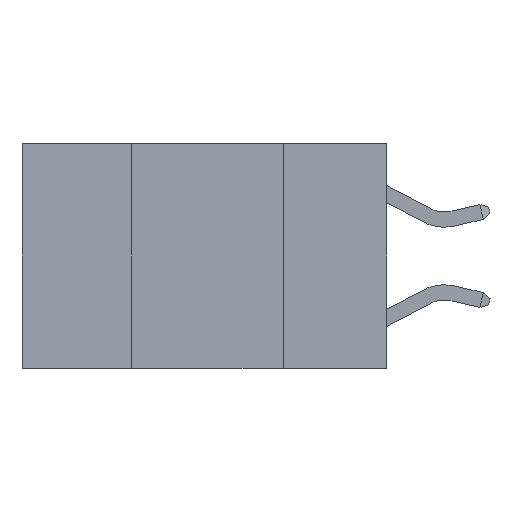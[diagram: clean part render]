
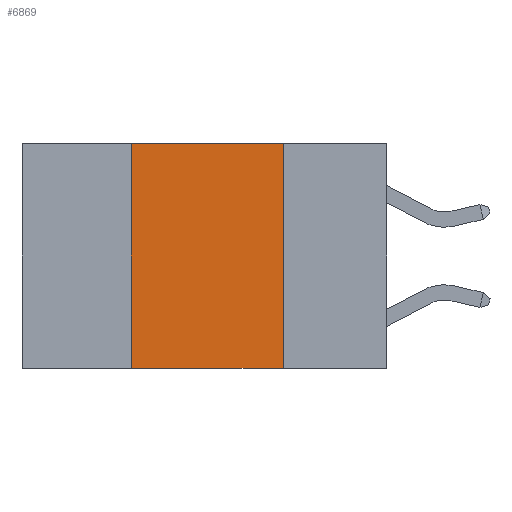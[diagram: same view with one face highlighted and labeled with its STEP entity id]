
A CAD part, left-side view. The second image highlights one B-rep face of the part: STEP entity #6869.
In plain terms, the highlighted planar face has unit normal (-1, 0, 0).
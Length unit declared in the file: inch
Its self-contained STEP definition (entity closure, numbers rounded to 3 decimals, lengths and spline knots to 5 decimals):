
#257 = FACE_OUTER_BOUND ( 'NONE', #26321, .T. ) ;
#2270 = LINE ( 'NONE', #10464, #5793 ) ;
#2395 = DIRECTION ( 'NONE',  ( 0., 0., -1. ) ) ;
#3506 = VECTOR ( 'NONE', #7858, 39.37008 ) ;
#3739 = EDGE_CURVE ( 'NONE', #3826, #25914, #2270, .T. ) ;
#3826 = VERTEX_POINT ( 'NONE', #24361 ) ;
#4052 = VERTEX_POINT ( 'NONE', #20062 ) ;
#4440 = DIRECTION ( 'NONE',  ( 0., 0., -1. ) ) ;
#5376 = CARTESIAN_POINT ( 'NONE',  ( 0., 0.42, 0. ) ) ;
#5665 = AXIS2_PLACEMENT_3D ( 'NONE', #24819, #14282, #4440 ) ;
#5793 = VECTOR ( 'NONE', #2395, 39.37008 ) ;
#6097 = ORIENTED_EDGE ( 'NONE', *, *, #3739, .F. ) ;
#6441 = PLANE ( 'NONE',  #5665 ) ;
#6869 = ADVANCED_FACE ( 'NONE', ( #257 ), #6441, .F. ) ;
#6937 = DIRECTION ( 'NONE',  ( 0., 0., 1. ) ) ;
#7195 = ORIENTED_EDGE ( 'NONE', *, *, #24867, .T. ) ;
#7238 = ORIENTED_EDGE ( 'NONE', *, *, #14618, .F. ) ;
#7858 = DIRECTION ( 'NONE',  ( 0., -1., 0. ) ) ;
#9956 = LINE ( 'NONE', #16432, #16304 ) ;
#10454 = LINE ( 'NONE', #16807, #25341 ) ;
#10464 = CARTESIAN_POINT ( 'NONE',  ( 0., 0.17, 0. ) ) ;
#11267 = VERTEX_POINT ( 'NONE', #5376 ) ;
#14282 = DIRECTION ( 'NONE',  ( 1., 0., 0. ) ) ;
#14618 = EDGE_CURVE ( 'NONE', #11267, #3826, #9956, .T. ) ;
#16304 = VECTOR ( 'NONE', #26580, 39.37008 ) ;
#16432 = CARTESIAN_POINT ( 'NONE',  ( 0., 0.6, 0. ) ) ;
#16807 = CARTESIAN_POINT ( 'NONE',  ( 0., 0.42, 0. ) ) ;
#18134 = LINE ( 'NONE', #20303, #3506 ) ;
#18793 = ORIENTED_EDGE ( 'NONE', *, *, #21188, .F. ) ;
#20062 = CARTESIAN_POINT ( 'NONE',  ( 0., 0.42, -0.37 ) ) ;
#20303 = CARTESIAN_POINT ( 'NONE',  ( 0., 0.6, -0.37 ) ) ;
#21188 = EDGE_CURVE ( 'NONE', #4052, #11267, #10454, .T. ) ;
#24291 = CARTESIAN_POINT ( 'NONE',  ( 0., 0.17, -0.37 ) ) ;
#24361 = CARTESIAN_POINT ( 'NONE',  ( 0., 0.17, 0. ) ) ;
#24819 = CARTESIAN_POINT ( 'NONE',  ( 0., 0.6, 0. ) ) ;
#24867 = EDGE_CURVE ( 'NONE', #4052, #25914, #18134, .T. ) ;
#25341 = VECTOR ( 'NONE', #6937, 39.37008 ) ;
#25914 = VERTEX_POINT ( 'NONE', #24291 ) ;
#26321 = EDGE_LOOP ( 'NONE', ( #6097, #7238, #18793, #7195 ) ) ;
#26580 = DIRECTION ( 'NONE',  ( 0., -1., 0. ) ) ;
